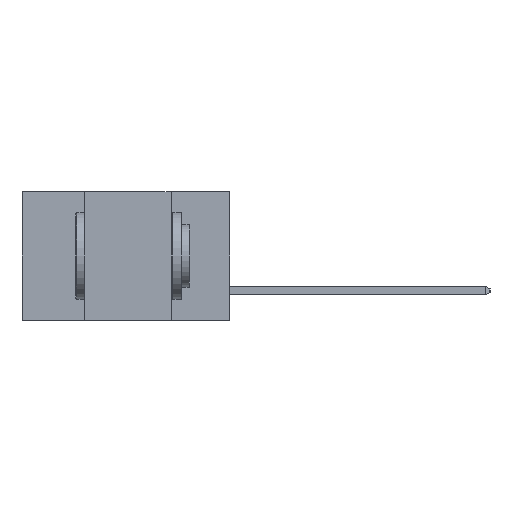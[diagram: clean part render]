
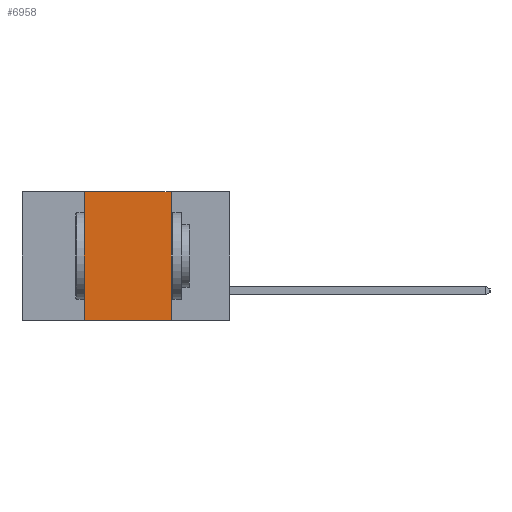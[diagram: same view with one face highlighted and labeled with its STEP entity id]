
A CAD part, left-side view. The second image highlights one B-rep face of the part: STEP entity #6958.
In plain terms, the highlighted planar face has unit normal (-1, 0, 0).
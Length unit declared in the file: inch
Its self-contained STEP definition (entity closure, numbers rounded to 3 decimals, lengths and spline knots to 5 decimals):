
#215 = CARTESIAN_POINT ( 'NONE',  ( 0., 0.17, -0.37 ) ) ;
#1686 = DIRECTION ( 'NONE',  ( 0., -1., 0. ) ) ;
#1755 = LINE ( 'NONE', #13735, #6374 ) ;
#3651 = FACE_OUTER_BOUND ( 'NONE', #15323, .T. ) ;
#5626 = ORIENTED_EDGE ( 'NONE', *, *, #7454, .F. ) ;
#5866 = PLANE ( 'NONE',  #15225 ) ;
#6040 = DIRECTION ( 'NONE',  ( 0., 0., 1. ) ) ;
#6374 = VECTOR ( 'NONE', #6040, 39.37008 ) ;
#6910 = VECTOR ( 'NONE', #24680, 39.37008 ) ;
#6958 = ADVANCED_FACE ( 'NONE', ( #3651 ), #5866, .F. ) ;
#7454 = EDGE_CURVE ( 'NONE', #19845, #10289, #7518, .T. ) ;
#7518 = LINE ( 'NONE', #13103, #6910 ) ;
#7792 = DIRECTION ( 'NONE',  ( 1., 0., 0. ) ) ;
#10289 = VERTEX_POINT ( 'NONE', #215 ) ;
#11492 = EDGE_CURVE ( 'NONE', #21811, #18423, #1755, .T. ) ;
#11644 = CARTESIAN_POINT ( 'NONE',  ( 0., 0.17, 0. ) ) ;
#12682 = CARTESIAN_POINT ( 'NONE',  ( 0., 0.42, 0. ) ) ;
#13103 = CARTESIAN_POINT ( 'NONE',  ( 0., 0.17, 0. ) ) ;
#13220 = EDGE_CURVE ( 'NONE', #18423, #19845, #16876, .T. ) ;
#13727 = DIRECTION ( 'NONE',  ( 0., -1., 0. ) ) ;
#13735 = CARTESIAN_POINT ( 'NONE',  ( 0., 0.42, 0. ) ) ;
#13768 = EDGE_CURVE ( 'NONE', #21811, #10289, #18601, .T. ) ;
#14711 = ORIENTED_EDGE ( 'NONE', *, *, #11492, .F. ) ;
#15225 = AXIS2_PLACEMENT_3D ( 'NONE', #19359, #7792, #21360 ) ;
#15323 = EDGE_LOOP ( 'NONE', ( #5626, #23779, #14711, #25272 ) ) ;
#16267 = VECTOR ( 'NONE', #13727, 39.37008 ) ;
#16876 = LINE ( 'NONE', #23399, #16267 ) ;
#17268 = CARTESIAN_POINT ( 'NONE',  ( 0., 0.6, -0.37 ) ) ;
#18423 = VERTEX_POINT ( 'NONE', #12682 ) ;
#18601 = LINE ( 'NONE', #17268, #23192 ) ;
#18990 = CARTESIAN_POINT ( 'NONE',  ( 0., 0.42, -0.37 ) ) ;
#19359 = CARTESIAN_POINT ( 'NONE',  ( 0., 0.6, 0. ) ) ;
#19845 = VERTEX_POINT ( 'NONE', #11644 ) ;
#21360 = DIRECTION ( 'NONE',  ( 0., 0., -1. ) ) ;
#21811 = VERTEX_POINT ( 'NONE', #18990 ) ;
#23192 = VECTOR ( 'NONE', #1686, 39.37008 ) ;
#23399 = CARTESIAN_POINT ( 'NONE',  ( 0., 0.6, 0. ) ) ;
#23779 = ORIENTED_EDGE ( 'NONE', *, *, #13220, .F. ) ;
#24680 = DIRECTION ( 'NONE',  ( 0., 0., -1. ) ) ;
#25272 = ORIENTED_EDGE ( 'NONE', *, *, #13768, .T. ) ;
